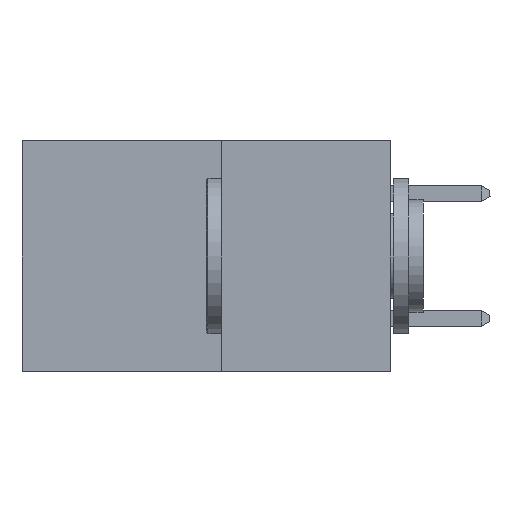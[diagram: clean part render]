
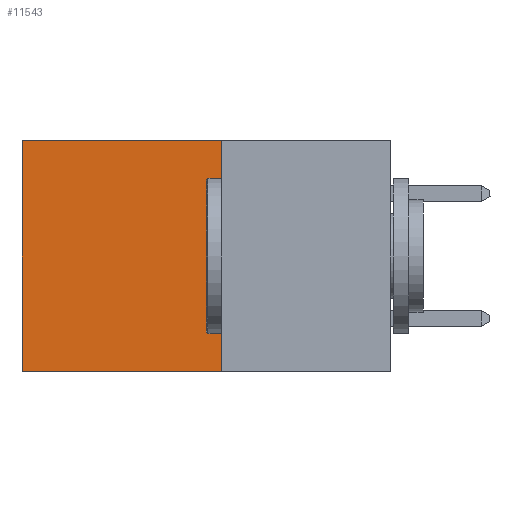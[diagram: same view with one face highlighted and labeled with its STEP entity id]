
A CAD part, left-side view. The second image highlights one B-rep face of the part: STEP entity #11543.
In plain terms, the highlighted planar face has unit normal (-1, 0, 0).
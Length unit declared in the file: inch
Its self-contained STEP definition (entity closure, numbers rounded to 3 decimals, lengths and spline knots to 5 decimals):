
#799 = ORIENTED_EDGE ( 'NONE', *, *, #16931, .F. ) ;
#968 = ORIENTED_EDGE ( 'NONE', *, *, #26700, .T. ) ;
#1411 = ORIENTED_EDGE ( 'NONE', *, *, #18411, .T. ) ;
#1658 = CARTESIAN_POINT ( 'NONE',  ( 0.277, 0.27, -0.37 ) ) ;
#2244 = CARTESIAN_POINT ( 'NONE',  ( 0.277, 0.59, -0.37 ) ) ;
#2276 = LINE ( 'NONE', #9531, #20100 ) ;
#2306 = VERTEX_POINT ( 'NONE', #2244 ) ;
#2660 = FACE_OUTER_BOUND ( 'NONE', #13407, .T. ) ;
#5807 = CARTESIAN_POINT ( 'NONE',  ( 0.277, 0.59, -0.37 ) ) ;
#5832 = CARTESIAN_POINT ( 'NONE',  ( 0.277, 0.27, -0.37 ) ) ;
#7179 = CARTESIAN_POINT ( 'NONE',  ( 0.277, 0.27, -0.37 ) ) ;
#8221 = DIRECTION ( 'NONE',  ( 0., 0., -1. ) ) ;
#8540 = LINE ( 'NONE', #1658, #13099 ) ;
#8733 = VERTEX_POINT ( 'NONE', #17242 ) ;
#9396 = DIRECTION ( 'NONE',  ( 1., 0., 0. ) ) ;
#9531 = CARTESIAN_POINT ( 'NONE',  ( 0.277, 0.27, -0.37 ) ) ;
#10258 = DIRECTION ( 'NONE',  ( 0., 0., -1. ) ) ;
#10494 = VECTOR ( 'NONE', #18440, 39.37008 ) ;
#11527 = VERTEX_POINT ( 'NONE', #27089 ) ;
#11543 = ADVANCED_FACE ( 'NONE', ( #2660 ), #20613, .F. ) ;
#11660 = ORIENTED_EDGE ( 'NONE', *, *, #15764, .F. ) ;
#13099 = VECTOR ( 'NONE', #8221, 39.37008 ) ;
#13407 = EDGE_LOOP ( 'NONE', ( #968, #799, #11660, #1411 ) ) ;
#13891 = CARTESIAN_POINT ( 'NONE',  ( 0.277, 0.27, 0. ) ) ;
#15764 = EDGE_CURVE ( 'NONE', #8733, #18008, #8540, .T. ) ;
#16931 = EDGE_CURVE ( 'NONE', #18008, #2306, #2276, .T. ) ;
#17242 = CARTESIAN_POINT ( 'NONE',  ( 0.277, 0.27, 0. ) ) ;
#18008 = VERTEX_POINT ( 'NONE', #5832 ) ;
#18411 = EDGE_CURVE ( 'NONE', #8733, #11527, #28163, .T. ) ;
#18440 = DIRECTION ( 'NONE',  ( 0., 1., 0. ) ) ;
#20100 = VECTOR ( 'NONE', #25177, 39.37008 ) ;
#20613 = PLANE ( 'NONE',  #23154 ) ;
#22534 = LINE ( 'NONE', #5807, #27533 ) ;
#23154 = AXIS2_PLACEMENT_3D ( 'NONE', #7179, #9396, #25049 ) ;
#25049 = DIRECTION ( 'NONE',  ( 0., 0., -1. ) ) ;
#25177 = DIRECTION ( 'NONE',  ( 0., 1., 0. ) ) ;
#26700 = EDGE_CURVE ( 'NONE', #11527, #2306, #22534, .T. ) ;
#27089 = CARTESIAN_POINT ( 'NONE',  ( 0.277, 0.59, 0. ) ) ;
#27533 = VECTOR ( 'NONE', #10258, 39.37008 ) ;
#28163 = LINE ( 'NONE', #13891, #10494 ) ;
